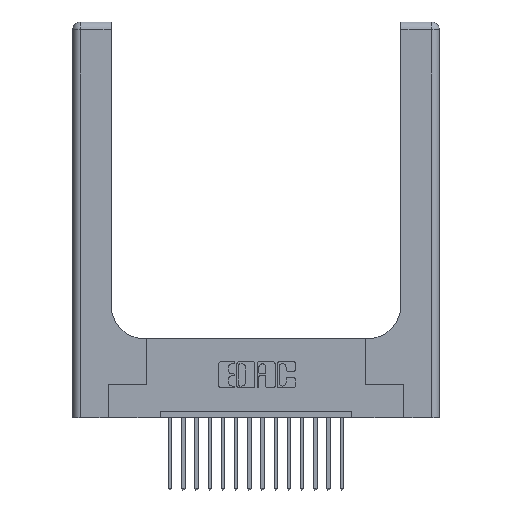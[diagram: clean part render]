
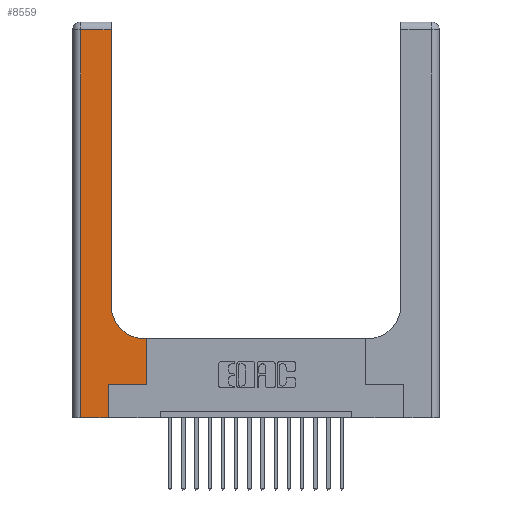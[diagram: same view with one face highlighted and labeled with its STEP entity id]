
A CAD part, top view. The second image highlights one B-rep face of the part: STEP entity #8559.
In plain terms, the highlighted planar face has unit normal (0, 0, 1).
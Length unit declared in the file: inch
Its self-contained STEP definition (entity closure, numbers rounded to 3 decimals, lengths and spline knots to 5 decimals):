
#345 = DIRECTION ( 'NONE',  ( 0., 0., -1. ) ) ;
#377 = DIRECTION ( 'NONE',  ( -1., 0., 0. ) ) ;
#407 = ORIENTED_EDGE ( 'NONE', *, *, #15667, .T. ) ;
#456 = EDGE_CURVE ( 'NONE', #13940, #16367, #3299, .T. ) ;
#1076 = VERTEX_POINT ( 'NONE', #18442 ) ;
#1281 = ORIENTED_EDGE ( 'NONE', *, *, #16832, .T. ) ;
#1377 = VECTOR ( 'NONE', #377, 39.37008 ) ;
#1433 = CARTESIAN_POINT ( 'NONE',  ( 0.06, 2.94, 0.37 ) ) ;
#1906 = CARTESIAN_POINT ( 'NONE',  ( 0.269, 0.25, 0.37 ) ) ;
#1925 = DIRECTION ( 'NONE',  ( 1., 0., 0. ) ) ;
#1934 = VECTOR ( 'NONE', #7109, 39.37008 ) ;
#2087 = CARTESIAN_POINT ( 'NONE',  ( 0.2915, 0.6, 0.37 ) ) ;
#2721 = CARTESIAN_POINT ( 'NONE',  ( 0.269, 0., 0.37 ) ) ;
#3061 = CARTESIAN_POINT ( 'NONE',  ( 0.06, 3., 0.37 ) ) ;
#3129 = EDGE_LOOP ( 'NONE', ( #17919, #10399, #1281, #17190, #8937, #9654, #7077, #3667, #407 ) ) ;
#3228 = CARTESIAN_POINT ( 'NONE',  ( 0.5415, 0.6, 0.37 ) ) ;
#3278 = CARTESIAN_POINT ( 'NONE',  ( 0., 3., 0.37 ) ) ;
#3299 = LINE ( 'NONE', #1906, #3559 ) ;
#3559 = VECTOR ( 'NONE', #16847, 39.37008 ) ;
#3667 = ORIENTED_EDGE ( 'NONE', *, *, #13034, .T. ) ;
#4030 = LINE ( 'NONE', #16127, #1934 ) ;
#4363 = DIRECTION ( 'NONE',  ( 0., -1., 0. ) ) ;
#4775 = CARTESIAN_POINT ( 'NONE',  ( 0.5585, 0.25, 0.37 ) ) ;
#4779 = DIRECTION ( 'NONE',  ( -1., 0., 0. ) ) ;
#4922 = CARTESIAN_POINT ( 'NONE',  ( 0.269, 0.25, 0.37 ) ) ;
#4966 = LINE ( 'NONE', #17452, #12978 ) ;
#6383 = VERTEX_POINT ( 'NONE', #12573 ) ;
#6453 = EDGE_CURVE ( 'NONE', #12386, #6383, #4966, .T. ) ;
#6508 = LINE ( 'NONE', #3061, #10016 ) ;
#7077 = ORIENTED_EDGE ( 'NONE', *, *, #9454, .T. ) ;
#7109 = DIRECTION ( 'NONE',  ( 0., 1., 0. ) ) ;
#7146 = LINE ( 'NONE', #18138, #13987 ) ;
#7775 = DIRECTION ( 'NONE',  ( 1., 0., 0. ) ) ;
#8559 = ADVANCED_FACE ( 'NONE', ( #18241 ), #16797, .F. ) ;
#8848 = LINE ( 'NONE', #11892, #14520 ) ;
#8937 = ORIENTED_EDGE ( 'NONE', *, *, #10442, .T. ) ;
#9339 = CARTESIAN_POINT ( 'NONE',  ( 0.5415, 0.85, 0.37 ) ) ;
#9454 = EDGE_CURVE ( 'NONE', #16367, #1076, #7146, .T. ) ;
#9654 = ORIENTED_EDGE ( 'NONE', *, *, #456, .T. ) ;
#10016 = VECTOR ( 'NONE', #4363, 39.37008 ) ;
#10143 = DIRECTION ( 'NONE',  ( 0., 1., 0. ) ) ;
#10399 = ORIENTED_EDGE ( 'NONE', *, *, #16282, .T. ) ;
#10442 = EDGE_CURVE ( 'NONE', #13356, #13940, #4030, .T. ) ;
#11036 = LINE ( 'NONE', #16799, #19049 ) ;
#11892 = CARTESIAN_POINT ( 'NONE',  ( 0., 2.94, 0.37 ) ) ;
#12126 = EDGE_CURVE ( 'NONE', #18980, #13356, #11036, .T. ) ;
#12386 = VERTEX_POINT ( 'NONE', #12625 ) ;
#12573 = CARTESIAN_POINT ( 'NONE',  ( 0.2915, 2.94, 0.37 ) ) ;
#12625 = CARTESIAN_POINT ( 'NONE',  ( 0.2915, 0.85, 0.37 ) ) ;
#12978 = VECTOR ( 'NONE', #10143, 39.37008 ) ;
#13034 = EDGE_CURVE ( 'NONE', #1076, #15082, #13616, .T. ) ;
#13287 = DIRECTION ( 'NONE',  ( -1., 0., 0. ) ) ;
#13356 = VERTEX_POINT ( 'NONE', #2721 ) ;
#13616 = LINE ( 'NONE', #2087, #1377 ) ;
#13823 = DIRECTION ( 'NONE',  ( 0., 0., -1. ) ) ;
#13940 = VERTEX_POINT ( 'NONE', #4922 ) ;
#13987 = VECTOR ( 'NONE', #16557, 39.37008 ) ;
#14520 = VECTOR ( 'NONE', #13287, 39.37008 ) ;
#15082 = VERTEX_POINT ( 'NONE', #3228 ) ;
#15667 = EDGE_CURVE ( 'NONE', #15082, #12386, #19260, .T. ) ;
#16127 = CARTESIAN_POINT ( 'NONE',  ( 0.269, 0., 0.37 ) ) ;
#16282 = EDGE_CURVE ( 'NONE', #6383, #18481, #8848, .T. ) ;
#16367 = VERTEX_POINT ( 'NONE', #4775 ) ;
#16557 = DIRECTION ( 'NONE',  ( 0., 1., 0. ) ) ;
#16797 = PLANE ( 'NONE',  #18317 ) ;
#16799 = CARTESIAN_POINT ( 'NONE',  ( 0., 0., 0.37 ) ) ;
#16832 = EDGE_CURVE ( 'NONE', #18481, #18980, #6508, .T. ) ;
#16847 = DIRECTION ( 'NONE',  ( 1., 0., 0. ) ) ;
#16894 = AXIS2_PLACEMENT_3D ( 'NONE', #9339, #345, #1925 ) ;
#17190 = ORIENTED_EDGE ( 'NONE', *, *, #12126, .T. ) ;
#17452 = CARTESIAN_POINT ( 'NONE',  ( 0.2915, 3., 0.37 ) ) ;
#17919 = ORIENTED_EDGE ( 'NONE', *, *, #6453, .T. ) ;
#18138 = CARTESIAN_POINT ( 'NONE',  ( 0.5585, 0.25, 0.37 ) ) ;
#18241 = FACE_OUTER_BOUND ( 'NONE', #3129, .T. ) ;
#18317 = AXIS2_PLACEMENT_3D ( 'NONE', #3278, #13823, #4779 ) ;
#18442 = CARTESIAN_POINT ( 'NONE',  ( 0.5585, 0.6, 0.37 ) ) ;
#18481 = VERTEX_POINT ( 'NONE', #1433 ) ;
#18980 = VERTEX_POINT ( 'NONE', #19214 ) ;
#19049 = VECTOR ( 'NONE', #7775, 39.37008 ) ;
#19214 = CARTESIAN_POINT ( 'NONE',  ( 0.06, 0., 0.37 ) ) ;
#19260 = CIRCLE ( 'NONE', #16894, 0.25 ) ;
